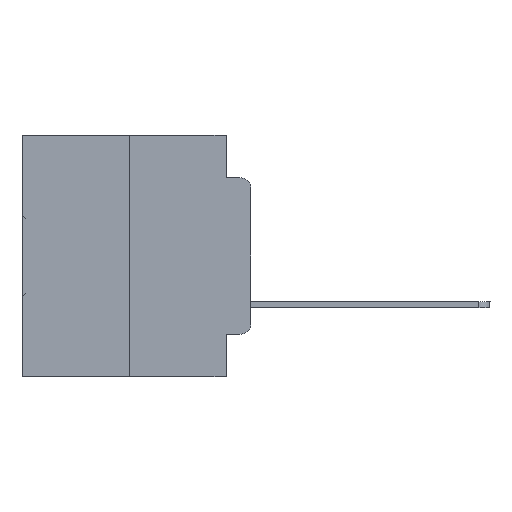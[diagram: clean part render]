
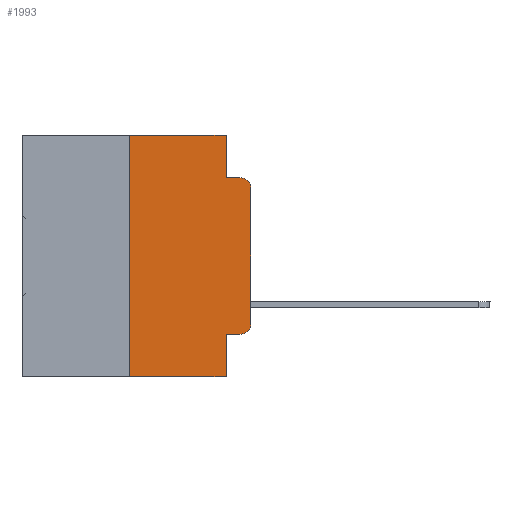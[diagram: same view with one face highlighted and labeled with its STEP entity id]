
A CAD part, left-side view. The second image highlights one B-rep face of the part: STEP entity #1993.
In plain terms, the highlighted planar face has unit normal (-1, 0, 0).
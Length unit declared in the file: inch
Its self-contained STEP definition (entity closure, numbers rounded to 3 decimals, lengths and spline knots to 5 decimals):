
#251 = DIRECTION ( 'NONE',  ( 0., -1., 0. ) ) ;
#546 = CARTESIAN_POINT ( 'NONE',  ( 0., 0.051, -0.0885 ) ) ;
#631 = EDGE_CURVE ( 'NONE', #12854, #12775, #32251, .T. ) ;
#825 = DIRECTION ( 'NONE',  ( 0., 0., -1. ) ) ;
#1026 = EDGE_CURVE ( 'NONE', #14434, #12775, #25692, .T. ) ;
#1177 = CARTESIAN_POINT ( 'NONE',  ( 0., 0.051, -0.5 ) ) ;
#1835 = CARTESIAN_POINT ( 'NONE',  ( 0., 0., -0.3915 ) ) ;
#1941 = CARTESIAN_POINT ( 'NONE',  ( 0., 0.02, -0.4115 ) ) ;
#1993 = ADVANCED_FACE ( 'NONE', ( #31784 ), #24607, .F. ) ;
#2305 = EDGE_LOOP ( 'NONE', ( #4089, #31259, #33566, #4047, #20799, #2840, #10760, #14674, #20180, #27158 ) ) ;
#2840 = ORIENTED_EDGE ( 'NONE', *, *, #14159, .F. ) ;
#2853 = VERTEX_POINT ( 'NONE', #3623 ) ;
#3530 = VECTOR ( 'NONE', #15437, 39.37008 ) ;
#3599 = DIRECTION ( 'NONE',  ( 1., 0., 0. ) ) ;
#3623 = CARTESIAN_POINT ( 'NONE',  ( 0., 0.25, 0. ) ) ;
#3704 = CARTESIAN_POINT ( 'NONE',  ( 0., 0.051, 0. ) ) ;
#3792 = DIRECTION ( 'NONE',  ( 0., -1., 0. ) ) ;
#4047 = ORIENTED_EDGE ( 'NONE', *, *, #21359, .F. ) ;
#4053 = VERTEX_POINT ( 'NONE', #26047 ) ;
#4089 = ORIENTED_EDGE ( 'NONE', *, *, #32182, .T. ) ;
#4742 = LINE ( 'NONE', #24612, #24961 ) ;
#5147 = CARTESIAN_POINT ( 'NONE',  ( 0., 0., 0. ) ) ;
#5171 = VECTOR ( 'NONE', #23485, 39.37008 ) ;
#5356 = CARTESIAN_POINT ( 'NONE',  ( 0., 0.25, -0.5 ) ) ;
#6134 = VECTOR ( 'NONE', #251, 39.37008 ) ;
#6936 = DIRECTION ( 'NONE',  ( 0., 0., -1. ) ) ;
#7354 = LINE ( 'NONE', #10888, #6134 ) ;
#8487 = LINE ( 'NONE', #9305, #11358 ) ;
#8904 = CARTESIAN_POINT ( 'NONE',  ( 0., 0.473, 0. ) ) ;
#9305 = CARTESIAN_POINT ( 'NONE',  ( 0., 0.473, 0. ) ) ;
#9455 = DIRECTION ( 'NONE',  ( -1., 0., 0. ) ) ;
#10136 = AXIS2_PLACEMENT_3D ( 'NONE', #8904, #3599, #22043 ) ;
#10760 = ORIENTED_EDGE ( 'NONE', *, *, #16243, .T. ) ;
#10888 = CARTESIAN_POINT ( 'NONE',  ( 0., 0.051, -0.4115 ) ) ;
#10896 = VERTEX_POINT ( 'NONE', #1835 ) ;
#11065 = EDGE_CURVE ( 'NONE', #31331, #10896, #12837, .T. ) ;
#11358 = VECTOR ( 'NONE', #32667, 39.37008 ) ;
#12775 = VERTEX_POINT ( 'NONE', #25417 ) ;
#12837 = CIRCLE ( 'NONE', #27982, 0.02 ) ;
#12854 = VERTEX_POINT ( 'NONE', #22848 ) ;
#13090 = DIRECTION ( 'NONE',  ( 0., 0., -1. ) ) ;
#13420 = CARTESIAN_POINT ( 'NONE',  ( 0., 0.02, -0.3915 ) ) ;
#14159 = EDGE_CURVE ( 'NONE', #15554, #2853, #33238, .T. ) ;
#14434 = VERTEX_POINT ( 'NONE', #546 ) ;
#14674 = ORIENTED_EDGE ( 'NONE', *, *, #24294, .F. ) ;
#15437 = DIRECTION ( 'NONE',  ( 0., 0., 1. ) ) ;
#15554 = VERTEX_POINT ( 'NONE', #5356 ) ;
#15568 = VERTEX_POINT ( 'NONE', #3704 ) ;
#16243 = EDGE_CURVE ( 'NONE', #15554, #25734, #20899, .T. ) ;
#16888 = EDGE_CURVE ( 'NONE', #2853, #15568, #8487, .T. ) ;
#17399 = DIRECTION ( 'NONE',  ( 0., -1., 0. ) ) ;
#20180 = ORIENTED_EDGE ( 'NONE', *, *, #32287, .T. ) ;
#20701 = VECTOR ( 'NONE', #17399, 39.37008 ) ;
#20799 = ORIENTED_EDGE ( 'NONE', *, *, #16888, .F. ) ;
#20899 = LINE ( 'NONE', #32709, #26267 ) ;
#20937 = CARTESIAN_POINT ( 'NONE',  ( 0., 0.051, 0. ) ) ;
#21359 = EDGE_CURVE ( 'NONE', #15568, #14434, #33200, .T. ) ;
#21803 = LINE ( 'NONE', #5147, #23068 ) ;
#22043 = DIRECTION ( 'NONE',  ( 0., 0., -1. ) ) ;
#22848 = CARTESIAN_POINT ( 'NONE',  ( 0., 0., -0.1085 ) ) ;
#23068 = VECTOR ( 'NONE', #29217, 39.37008 ) ;
#23485 = DIRECTION ( 'NONE',  ( 0., 0., -1. ) ) ;
#23845 = DIRECTION ( 'NONE',  ( -1., 0., 0. ) ) ;
#24294 = EDGE_CURVE ( 'NONE', #4053, #25734, #4742, .T. ) ;
#24607 = PLANE ( 'NONE',  #10136 ) ;
#24612 = CARTESIAN_POINT ( 'NONE',  ( 0., 0.051, 0. ) ) ;
#24961 = VECTOR ( 'NONE', #825, 39.37008 ) ;
#25417 = CARTESIAN_POINT ( 'NONE',  ( 0., 0.02, -0.0885 ) ) ;
#25692 = LINE ( 'NONE', #30985, #20701 ) ;
#25734 = VERTEX_POINT ( 'NONE', #1177 ) ;
#26047 = CARTESIAN_POINT ( 'NONE',  ( 0., 0.051, -0.4115 ) ) ;
#26267 = VECTOR ( 'NONE', #3792, 39.37008 ) ;
#27158 = ORIENTED_EDGE ( 'NONE', *, *, #11065, .T. ) ;
#27571 = AXIS2_PLACEMENT_3D ( 'NONE', #30088, #9455, #6936 ) ;
#27982 = AXIS2_PLACEMENT_3D ( 'NONE', #13420, #23845, #13090 ) ;
#29217 = DIRECTION ( 'NONE',  ( 0., 0., 1. ) ) ;
#30088 = CARTESIAN_POINT ( 'NONE',  ( 0., 0.02, -0.1085 ) ) ;
#30985 = CARTESIAN_POINT ( 'NONE',  ( 0., 0.051, -0.0885 ) ) ;
#30997 = CARTESIAN_POINT ( 'NONE',  ( 0., 0.25, 0. ) ) ;
#31259 = ORIENTED_EDGE ( 'NONE', *, *, #631, .T. ) ;
#31331 = VERTEX_POINT ( 'NONE', #1941 ) ;
#31784 = FACE_OUTER_BOUND ( 'NONE', #2305, .T. ) ;
#32182 = EDGE_CURVE ( 'NONE', #10896, #12854, #21803, .T. ) ;
#32251 = CIRCLE ( 'NONE', #27571, 0.02 ) ;
#32287 = EDGE_CURVE ( 'NONE', #4053, #31331, #7354, .T. ) ;
#32667 = DIRECTION ( 'NONE',  ( 0., -1., 0. ) ) ;
#32709 = CARTESIAN_POINT ( 'NONE',  ( 0., 0.473, -0.5 ) ) ;
#33200 = LINE ( 'NONE', #20937, #5171 ) ;
#33238 = LINE ( 'NONE', #30997, #3530 ) ;
#33566 = ORIENTED_EDGE ( 'NONE', *, *, #1026, .F. ) ;
